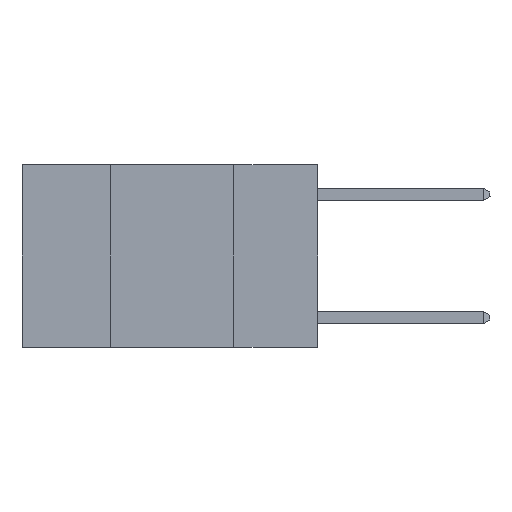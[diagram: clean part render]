
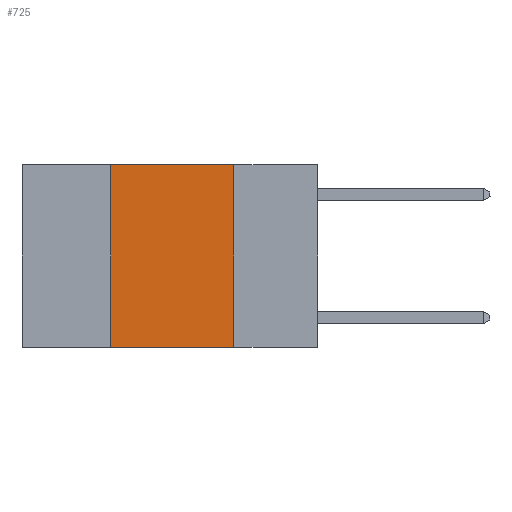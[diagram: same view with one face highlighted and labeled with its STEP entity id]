
A CAD part, left-side view. The second image highlights one B-rep face of the part: STEP entity #725.
In plain terms, the highlighted planar face has unit normal (-1, 0, 0).
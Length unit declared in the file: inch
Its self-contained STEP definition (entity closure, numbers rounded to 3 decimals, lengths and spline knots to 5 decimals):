
#725 = ADVANCED_FACE ( 'NONE', ( #1231 ), #5816, .F. ) ;
#1231 = FACE_OUTER_BOUND ( 'NONE', #22132, .T. ) ;
#1840 = ORIENTED_EDGE ( 'NONE', *, *, #5552, .F. ) ;
#2403 = EDGE_CURVE ( 'NONE', #2945, #15894, #17386, .T. ) ;
#2945 = VERTEX_POINT ( 'NONE', #20362 ) ;
#4225 = ORIENTED_EDGE ( 'NONE', *, *, #24927, .T. ) ;
#4254 = VECTOR ( 'NONE', #11469, 39.37008 ) ;
#5425 = CARTESIAN_POINT ( 'NONE',  ( 0., 0.17, -0.37 ) ) ;
#5552 = EDGE_CURVE ( 'NONE', #15610, #10023, #11191, .T. ) ;
#5681 = DIRECTION ( 'NONE',  ( 0., 0., -1. ) ) ;
#5816 = PLANE ( 'NONE',  #17132 ) ;
#5977 = DIRECTION ( 'NONE',  ( 0., -1., 0. ) ) ;
#9038 = DIRECTION ( 'NONE',  ( 0., 0., -1. ) ) ;
#10023 = VERTEX_POINT ( 'NONE', #26840 ) ;
#11109 = DIRECTION ( 'NONE',  ( 0., -1., 0. ) ) ;
#11191 = LINE ( 'NONE', #24164, #4254 ) ;
#11393 = CARTESIAN_POINT ( 'NONE',  ( 0., 0.17, 0. ) ) ;
#11469 = DIRECTION ( 'NONE',  ( 0., 0., 1. ) ) ;
#12041 = VECTOR ( 'NONE', #5977, 39.37008 ) ;
#12213 = CARTESIAN_POINT ( 'NONE',  ( 0., 0.6, 0. ) ) ;
#13318 = VECTOR ( 'NONE', #11109, 39.37008 ) ;
#14578 = DIRECTION ( 'NONE',  ( 1., 0., 0. ) ) ;
#15311 = CARTESIAN_POINT ( 'NONE',  ( 0., 0.42, -0.37 ) ) ;
#15610 = VERTEX_POINT ( 'NONE', #15311 ) ;
#15764 = ORIENTED_EDGE ( 'NONE', *, *, #26688, .F. ) ;
#15894 = VERTEX_POINT ( 'NONE', #5425 ) ;
#16153 = CARTESIAN_POINT ( 'NONE',  ( 0., 0.6, 0. ) ) ;
#17132 = AXIS2_PLACEMENT_3D ( 'NONE', #12213, #14578, #5681 ) ;
#17244 = LINE ( 'NONE', #19444, #13318 ) ;
#17386 = LINE ( 'NONE', #11393, #19857 ) ;
#19444 = CARTESIAN_POINT ( 'NONE',  ( 0., 0.6, -0.37 ) ) ;
#19857 = VECTOR ( 'NONE', #9038, 39.37008 ) ;
#20362 = CARTESIAN_POINT ( 'NONE',  ( 0., 0.17, 0. ) ) ;
#20740 = LINE ( 'NONE', #16153, #12041 ) ;
#22132 = EDGE_LOOP ( 'NONE', ( #26499, #15764, #1840, #4225 ) ) ;
#24164 = CARTESIAN_POINT ( 'NONE',  ( 0., 0.42, 0. ) ) ;
#24927 = EDGE_CURVE ( 'NONE', #15610, #15894, #17244, .T. ) ;
#26499 = ORIENTED_EDGE ( 'NONE', *, *, #2403, .F. ) ;
#26688 = EDGE_CURVE ( 'NONE', #10023, #2945, #20740, .T. ) ;
#26840 = CARTESIAN_POINT ( 'NONE',  ( 0., 0.42, 0. ) ) ;
